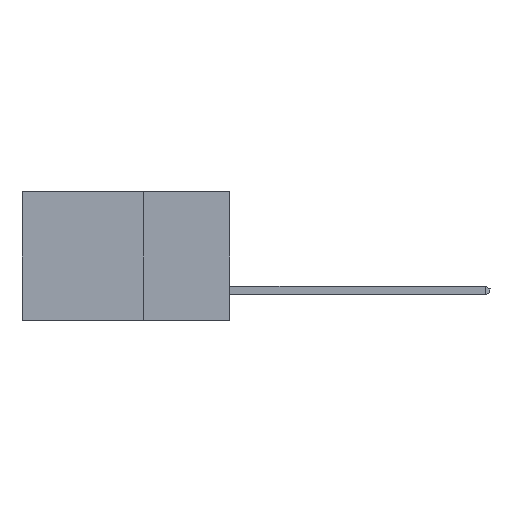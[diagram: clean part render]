
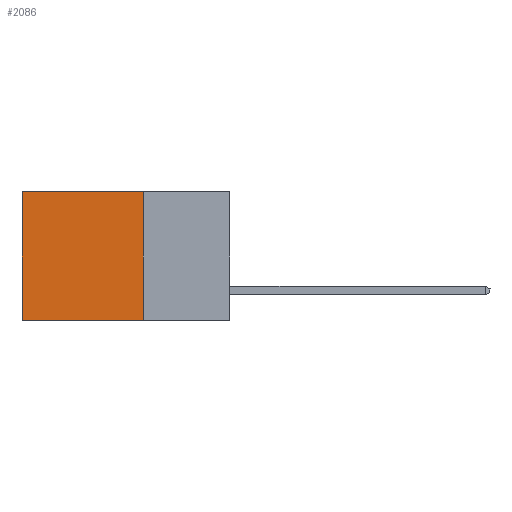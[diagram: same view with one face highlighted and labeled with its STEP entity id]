
A CAD part, left-side view. The second image highlights one B-rep face of the part: STEP entity #2086.
In plain terms, the highlighted planar face has unit normal (-1, 0, 0).
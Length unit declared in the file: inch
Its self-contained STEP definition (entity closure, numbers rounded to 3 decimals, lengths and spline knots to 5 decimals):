
#300 = EDGE_CURVE ( 'NONE', #754, #10370, #9761, .T. ) ;
#307 = DIRECTION ( 'NONE',  ( 0., 0., -1. ) ) ;
#754 = VERTEX_POINT ( 'NONE', #1241 ) ;
#1241 = CARTESIAN_POINT ( 'NONE',  ( 0.2615, 0.25, -0.37 ) ) ;
#1281 = VECTOR ( 'NONE', #3520, 39.37008 ) ;
#1463 = EDGE_CURVE ( 'NONE', #3728, #10370, #14519, .T. ) ;
#1472 = ORIENTED_EDGE ( 'NONE', *, *, #7430, .F. ) ;
#1487 = FACE_OUTER_BOUND ( 'NONE', #5868, .T. ) ;
#2026 = DIRECTION ( 'NONE',  ( 1., 0., 0. ) ) ;
#2086 = ADVANCED_FACE ( 'NONE', ( #1487 ), #6371, .F. ) ;
#3217 = CARTESIAN_POINT ( 'NONE',  ( 0.2615, 0.6, -0.37 ) ) ;
#3520 = DIRECTION ( 'NONE',  ( 0., 1., 0. ) ) ;
#3728 = VERTEX_POINT ( 'NONE', #4352 ) ;
#3925 = DIRECTION ( 'NONE',  ( 0., 1., 0. ) ) ;
#4352 = CARTESIAN_POINT ( 'NONE',  ( 0.2615, 0.6, 0. ) ) ;
#4445 = CARTESIAN_POINT ( 'NONE',  ( 0.2615, 0.25, -0.37 ) ) ;
#5794 = EDGE_CURVE ( 'NONE', #12251, #3728, #11045, .T. ) ;
#5868 = EDGE_LOOP ( 'NONE', ( #5904, #8846, #1472, #13389 ) ) ;
#5904 = ORIENTED_EDGE ( 'NONE', *, *, #1463, .T. ) ;
#6239 = CARTESIAN_POINT ( 'NONE',  ( 0.2615, 0.25, 0. ) ) ;
#6270 = VECTOR ( 'NONE', #307, 39.37008 ) ;
#6345 = CARTESIAN_POINT ( 'NONE',  ( 0.2615, 0.6, -0.37 ) ) ;
#6371 = PLANE ( 'NONE',  #7986 ) ;
#7430 = EDGE_CURVE ( 'NONE', #12251, #754, #7617, .T. ) ;
#7617 = LINE ( 'NONE', #11311, #6270 ) ;
#7986 = AXIS2_PLACEMENT_3D ( 'NONE', #4445, #2026, #13908 ) ;
#8118 = VECTOR ( 'NONE', #3925, 39.37008 ) ;
#8846 = ORIENTED_EDGE ( 'NONE', *, *, #300, .F. ) ;
#9761 = LINE ( 'NONE', #14651, #1281 ) ;
#10267 = CARTESIAN_POINT ( 'NONE',  ( 0.2615, 0.25, 0. ) ) ;
#10370 = VERTEX_POINT ( 'NONE', #6345 ) ;
#11045 = LINE ( 'NONE', #6239, #8118 ) ;
#11311 = CARTESIAN_POINT ( 'NONE',  ( 0.2615, 0.25, -0.37 ) ) ;
#12251 = VERTEX_POINT ( 'NONE', #10267 ) ;
#13161 = DIRECTION ( 'NONE',  ( 0., 0., -1. ) ) ;
#13389 = ORIENTED_EDGE ( 'NONE', *, *, #5794, .T. ) ;
#13908 = DIRECTION ( 'NONE',  ( 0., 0., -1. ) ) ;
#14519 = LINE ( 'NONE', #3217, #15136 ) ;
#14651 = CARTESIAN_POINT ( 'NONE',  ( 0.2615, 0.25, -0.37 ) ) ;
#15136 = VECTOR ( 'NONE', #13161, 39.37008 ) ;
